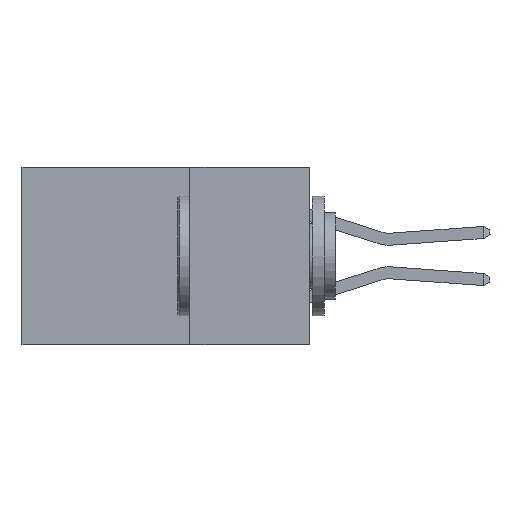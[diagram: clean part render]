
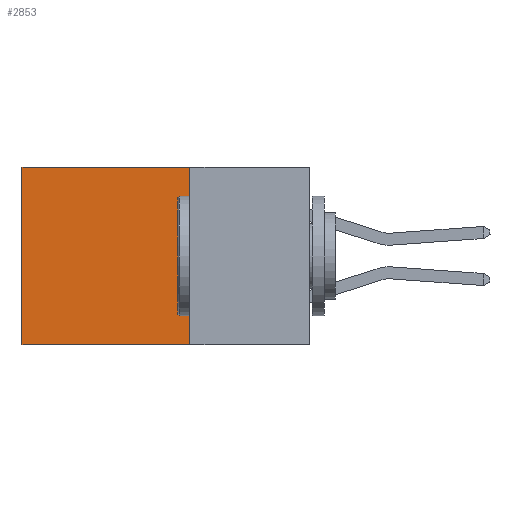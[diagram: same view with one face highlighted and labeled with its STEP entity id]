
A CAD part, left-side view. The second image highlights one B-rep face of the part: STEP entity #2853.
In plain terms, the highlighted planar face has unit normal (-1, 0, 0).
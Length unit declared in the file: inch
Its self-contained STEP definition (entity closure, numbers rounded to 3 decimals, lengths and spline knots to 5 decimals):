
#759 = CARTESIAN_POINT ( 'NONE',  ( 0.2615, 0.25, -0.37 ) ) ;
#786 = DIRECTION ( 'NONE',  ( 0., 1., 0. ) ) ;
#1007 = LINE ( 'NONE', #3127, #8439 ) ;
#1573 = DIRECTION ( 'NONE',  ( 0., 0., -1. ) ) ;
#1598 = DIRECTION ( 'NONE',  ( 1., 0., 0. ) ) ;
#1752 = CARTESIAN_POINT ( 'NONE',  ( 0.2615, 0.25, -0.37 ) ) ;
#1887 = VERTEX_POINT ( 'NONE', #5459 ) ;
#2244 = VERTEX_POINT ( 'NONE', #10722 ) ;
#2350 = PLANE ( 'NONE',  #8831 ) ;
#2853 = ADVANCED_FACE ( 'NONE', ( #4603 ), #2350, .F. ) ;
#3011 = DIRECTION ( 'NONE',  ( 0., 1., 0. ) ) ;
#3127 = CARTESIAN_POINT ( 'NONE',  ( 0.2615, 0.25, 0. ) ) ;
#3244 = VERTEX_POINT ( 'NONE', #6149 ) ;
#3627 = EDGE_CURVE ( 'NONE', #2244, #5670, #9759, .T. ) ;
#4009 = VECTOR ( 'NONE', #11471, 39.37008 ) ;
#4603 = FACE_OUTER_BOUND ( 'NONE', #5226, .T. ) ;
#4770 = ORIENTED_EDGE ( 'NONE', *, *, #8327, .F. ) ;
#4811 = EDGE_CURVE ( 'NONE', #3244, #2244, #1007, .T. ) ;
#5226 = EDGE_LOOP ( 'NONE', ( #8974, #4770, #11766, #11317 ) ) ;
#5459 = CARTESIAN_POINT ( 'NONE',  ( 0.2615, 0.25, -0.37 ) ) ;
#5670 = VERTEX_POINT ( 'NONE', #12008 ) ;
#6149 = CARTESIAN_POINT ( 'NONE',  ( 0.2615, 0.25, 0. ) ) ;
#8327 = EDGE_CURVE ( 'NONE', #1887, #5670, #10356, .T. ) ;
#8439 = VECTOR ( 'NONE', #3011, 39.37008 ) ;
#8831 = AXIS2_PLACEMENT_3D ( 'NONE', #1752, #1598, #1573 ) ;
#8974 = ORIENTED_EDGE ( 'NONE', *, *, #3627, .T. ) ;
#9000 = EDGE_CURVE ( 'NONE', #3244, #1887, #9049, .T. ) ;
#9049 = LINE ( 'NONE', #11540, #4009 ) ;
#9759 = LINE ( 'NONE', #11707, #11653 ) ;
#10062 = VECTOR ( 'NONE', #786, 39.37008 ) ;
#10356 = LINE ( 'NONE', #759, #10062 ) ;
#10722 = CARTESIAN_POINT ( 'NONE',  ( 0.2615, 0.6, 0. ) ) ;
#11317 = ORIENTED_EDGE ( 'NONE', *, *, #4811, .T. ) ;
#11471 = DIRECTION ( 'NONE',  ( 0., 0., -1. ) ) ;
#11540 = CARTESIAN_POINT ( 'NONE',  ( 0.2615, 0.25, -0.37 ) ) ;
#11653 = VECTOR ( 'NONE', #11683, 39.37008 ) ;
#11683 = DIRECTION ( 'NONE',  ( 0., 0., -1. ) ) ;
#11707 = CARTESIAN_POINT ( 'NONE',  ( 0.2615, 0.6, -0.37 ) ) ;
#11766 = ORIENTED_EDGE ( 'NONE', *, *, #9000, .F. ) ;
#12008 = CARTESIAN_POINT ( 'NONE',  ( 0.2615, 0.6, -0.37 ) ) ;
